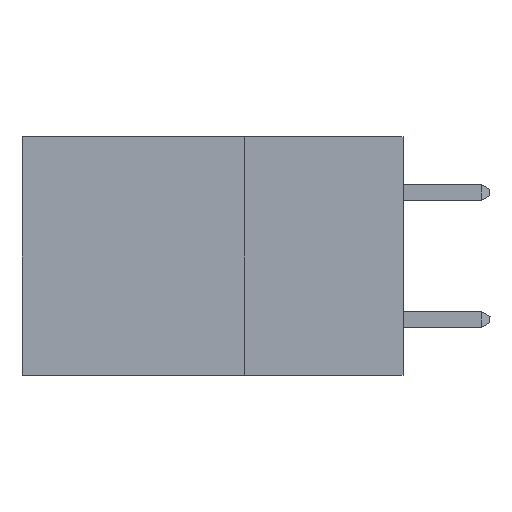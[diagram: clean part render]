
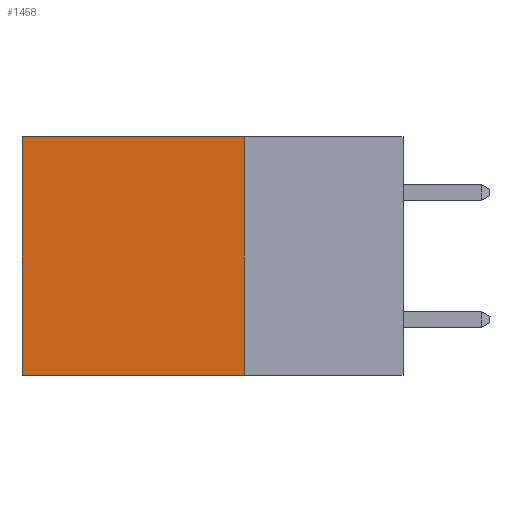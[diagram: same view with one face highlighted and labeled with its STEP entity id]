
A CAD part, left-side view. The second image highlights one B-rep face of the part: STEP entity #1458.
In plain terms, the highlighted planar face has unit normal (-1, 0, 0).
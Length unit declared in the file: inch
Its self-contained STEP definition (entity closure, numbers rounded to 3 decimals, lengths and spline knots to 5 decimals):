
#1458 = ADVANCED_FACE ( 'NONE', ( #9216 ), #17887, .F. ) ;
#1571 = CARTESIAN_POINT ( 'NONE',  ( 0.2875, 0.25, 0. ) ) ;
#1917 = CARTESIAN_POINT ( 'NONE',  ( 0.2875, 0.6, -0.375 ) ) ;
#2580 = CARTESIAN_POINT ( 'NONE',  ( 0.2875, 0.25, -0.375 ) ) ;
#3184 = VERTEX_POINT ( 'NONE', #1571 ) ;
#3272 = EDGE_CURVE ( 'NONE', #3184, #16928, #15742, .T. ) ;
#3765 = LINE ( 'NONE', #20329, #16743 ) ;
#4044 = DIRECTION ( 'NONE',  ( 0., 0., -1. ) ) ;
#4218 = DIRECTION ( 'NONE',  ( 0., 0., -1. ) ) ;
#5111 = EDGE_CURVE ( 'NONE', #16928, #6171, #9080, .T. ) ;
#5350 = DIRECTION ( 'NONE',  ( 0., 1., 0. ) ) ;
#5427 = CARTESIAN_POINT ( 'NONE',  ( 0.2875, 0.6, 0. ) ) ;
#6171 = VERTEX_POINT ( 'NONE', #1917 ) ;
#6558 = VECTOR ( 'NONE', #4218, 39.37008 ) ;
#7767 = DIRECTION ( 'NONE',  ( 0., 0., -1. ) ) ;
#7920 = CARTESIAN_POINT ( 'NONE',  ( 0.2875, 0.25, -0.375 ) ) ;
#8025 = ORIENTED_EDGE ( 'NONE', *, *, #5111, .T. ) ;
#9080 = LINE ( 'NONE', #13515, #19078 ) ;
#9216 = FACE_OUTER_BOUND ( 'NONE', #19646, .T. ) ;
#9346 = DIRECTION ( 'NONE',  ( 1., 0., 0. ) ) ;
#9400 = ORIENTED_EDGE ( 'NONE', *, *, #10324, .F. ) ;
#9528 = CARTESIAN_POINT ( 'NONE',  ( 0.2875, 0.25, -0.375 ) ) ;
#9835 = VERTEX_POINT ( 'NONE', #9528 ) ;
#10221 = DIRECTION ( 'NONE',  ( 0., 1., 0. ) ) ;
#10324 = EDGE_CURVE ( 'NONE', #3184, #9835, #15572, .T. ) ;
#11283 = VECTOR ( 'NONE', #10221, 39.37008 ) ;
#13515 = CARTESIAN_POINT ( 'NONE',  ( 0.2875, 0.6, -0.375 ) ) ;
#15325 = ORIENTED_EDGE ( 'NONE', *, *, #17831, .F. ) ;
#15572 = LINE ( 'NONE', #7920, #6558 ) ;
#15742 = LINE ( 'NONE', #18429, #11283 ) ;
#16743 = VECTOR ( 'NONE', #5350, 39.37008 ) ;
#16928 = VERTEX_POINT ( 'NONE', #5427 ) ;
#17831 = EDGE_CURVE ( 'NONE', #9835, #6171, #3765, .T. ) ;
#17887 = PLANE ( 'NONE',  #20763 ) ;
#18429 = CARTESIAN_POINT ( 'NONE',  ( 0.2875, 0.25, 0. ) ) ;
#19078 = VECTOR ( 'NONE', #4044, 39.37008 ) ;
#19370 = ORIENTED_EDGE ( 'NONE', *, *, #3272, .T. ) ;
#19646 = EDGE_LOOP ( 'NONE', ( #8025, #15325, #9400, #19370 ) ) ;
#20329 = CARTESIAN_POINT ( 'NONE',  ( 0.2875, 0.25, -0.375 ) ) ;
#20763 = AXIS2_PLACEMENT_3D ( 'NONE', #2580, #9346, #7767 ) ;
